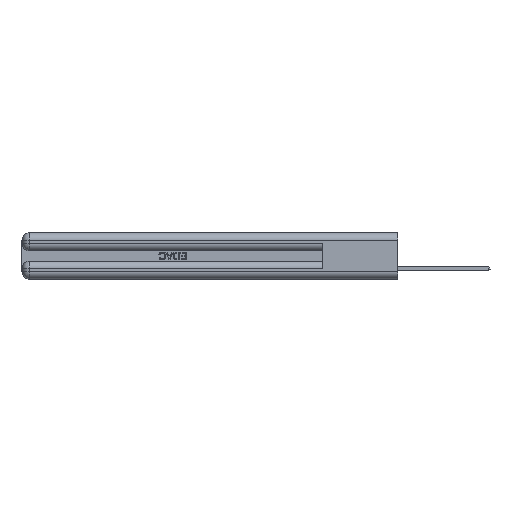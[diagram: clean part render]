
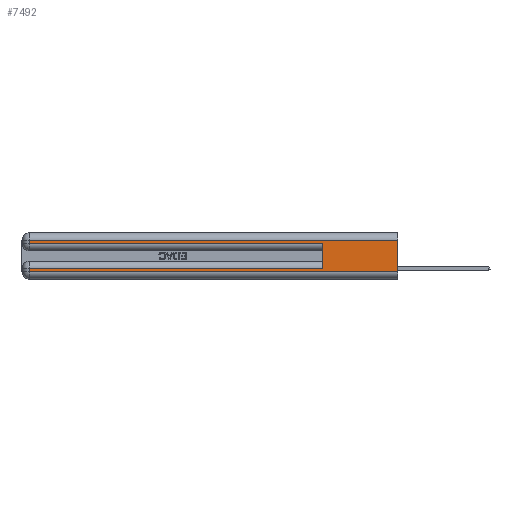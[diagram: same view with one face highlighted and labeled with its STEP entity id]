
A CAD part, left-side view. The second image highlights one B-rep face of the part: STEP entity #7492.
In plain terms, the highlighted planar face has unit normal (-1, 0, 0).
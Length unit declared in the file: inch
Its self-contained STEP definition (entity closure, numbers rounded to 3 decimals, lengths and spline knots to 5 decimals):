
#1328 = VERTEX_POINT ( 'NONE', #38254 ) ;
#1911 = VECTOR ( 'NONE', #44881, 39.37008 ) ;
#5257 = EDGE_CURVE ( 'NONE', #1328, #14109, #14674, .T. ) ;
#5522 = VERTEX_POINT ( 'NONE', #23589 ) ;
#5828 = CARTESIAN_POINT ( 'NONE',  ( 0., 2.94, 0.31 ) ) ;
#6140 = CARTESIAN_POINT ( 'NONE',  ( 0., 0., 0.37 ) ) ;
#7248 = LINE ( 'NONE', #36885, #1911 ) ;
#7492 = ADVANCED_FACE ( 'NONE', ( #13577 ), #10854, .F. ) ;
#7686 = LINE ( 'NONE', #51224, #41666 ) ;
#7776 = VERTEX_POINT ( 'NONE', #51697 ) ;
#8434 = ORIENTED_EDGE ( 'NONE', *, *, #53814, .T. ) ;
#10840 = LINE ( 'NONE', #38863, #15516 ) ;
#10854 = PLANE ( 'NONE',  #31321 ) ;
#11121 = CARTESIAN_POINT ( 'NONE',  ( 0., 0., 0.31 ) ) ;
#11753 = ORIENTED_EDGE ( 'NONE', *, *, #25905, .F. ) ;
#13577 = FACE_OUTER_BOUND ( 'NONE', #14585, .T. ) ;
#14109 = VERTEX_POINT ( 'NONE', #25756 ) ;
#14332 = VECTOR ( 'NONE', #20107, 39.37008 ) ;
#14585 = EDGE_LOOP ( 'NONE', ( #11753, #47032, #16410, #8434, #43683, #26335, #26392, #51709 ) ) ;
#14674 = LINE ( 'NONE', #42219, #18711 ) ;
#15516 = VECTOR ( 'NONE', #30175, 39.37008 ) ;
#16410 = ORIENTED_EDGE ( 'NONE', *, *, #35955, .T. ) ;
#18711 = VECTOR ( 'NONE', #28849, 39.37008 ) ;
#20107 = DIRECTION ( 'NONE',  ( 0., 1., 0. ) ) ;
#21126 = VECTOR ( 'NONE', #30723, 39.37008 ) ;
#21949 = EDGE_CURVE ( 'NONE', #5522, #31353, #50923, .T. ) ;
#22140 = CARTESIAN_POINT ( 'NONE',  ( 0., 0., 0.06 ) ) ;
#22474 = LINE ( 'NONE', #22140, #21126 ) ;
#23235 = CARTESIAN_POINT ( 'NONE',  ( 0., 2.94, 0.06 ) ) ;
#23589 = CARTESIAN_POINT ( 'NONE',  ( 0., 0., 0.31 ) ) ;
#23928 = DIRECTION ( 'NONE',  ( 1., 0., 0. ) ) ;
#25288 = DIRECTION ( 'NONE',  ( 0., 0., -1. ) ) ;
#25756 = CARTESIAN_POINT ( 'NONE',  ( 0., 2.94, 0.085 ) ) ;
#25905 = EDGE_CURVE ( 'NONE', #5522, #35526, #33705, .T. ) ;
#26335 = ORIENTED_EDGE ( 'NONE', *, *, #5257, .T. ) ;
#26392 = ORIENTED_EDGE ( 'NONE', *, *, #52669, .T. ) ;
#28421 = CARTESIAN_POINT ( 'NONE',  ( 0., 0., 0.06 ) ) ;
#28849 = DIRECTION ( 'NONE',  ( 0., 1., 0. ) ) ;
#30175 = DIRECTION ( 'NONE',  ( 0., -1., 0. ) ) ;
#30723 = DIRECTION ( 'NONE',  ( 0., -1., 0. ) ) ;
#31321 = AXIS2_PLACEMENT_3D ( 'NONE', #41568, #23928, #47312 ) ;
#31353 = VERTEX_POINT ( 'NONE', #5828 ) ;
#31973 = VERTEX_POINT ( 'NONE', #23235 ) ;
#32733 = DIRECTION ( 'NONE',  ( 0., 0., 1. ) ) ;
#33705 = LINE ( 'NONE', #6140, #44384 ) ;
#33746 = LINE ( 'NONE', #49228, #54985 ) ;
#35526 = VERTEX_POINT ( 'NONE', #28421 ) ;
#35955 = EDGE_CURVE ( 'NONE', #31353, #7776, #7248, .T. ) ;
#36622 = VERTEX_POINT ( 'NONE', #45545 ) ;
#36885 = CARTESIAN_POINT ( 'NONE',  ( 0., 2.94, 0.37 ) ) ;
#38254 = CARTESIAN_POINT ( 'NONE',  ( 0., 0.6, 0.085 ) ) ;
#38863 = CARTESIAN_POINT ( 'NONE',  ( 0., 0., 0.285 ) ) ;
#39271 = EDGE_CURVE ( 'NONE', #31973, #35526, #22474, .T. ) ;
#39533 = EDGE_CURVE ( 'NONE', #1328, #36622, #33746, .T. ) ;
#41568 = CARTESIAN_POINT ( 'NONE',  ( 0., 0., 0.37 ) ) ;
#41666 = VECTOR ( 'NONE', #25288, 39.37008 ) ;
#42219 = CARTESIAN_POINT ( 'NONE',  ( 0., 0., 0.085 ) ) ;
#43683 = ORIENTED_EDGE ( 'NONE', *, *, #39533, .F. ) ;
#44384 = VECTOR ( 'NONE', #48205, 39.37008 ) ;
#44881 = DIRECTION ( 'NONE',  ( 0., 0., -1. ) ) ;
#45545 = CARTESIAN_POINT ( 'NONE',  ( 0., 0.6, 0.285 ) ) ;
#47032 = ORIENTED_EDGE ( 'NONE', *, *, #21949, .T. ) ;
#47312 = DIRECTION ( 'NONE',  ( 0., 0., -1. ) ) ;
#48205 = DIRECTION ( 'NONE',  ( 0., 0., -1. ) ) ;
#49228 = CARTESIAN_POINT ( 'NONE',  ( 0., 0.6, 0.145 ) ) ;
#50923 = LINE ( 'NONE', #11121, #14332 ) ;
#51224 = CARTESIAN_POINT ( 'NONE',  ( 0., 2.94, 0.37 ) ) ;
#51697 = CARTESIAN_POINT ( 'NONE',  ( 0., 2.94, 0.285 ) ) ;
#51709 = ORIENTED_EDGE ( 'NONE', *, *, #39271, .T. ) ;
#52669 = EDGE_CURVE ( 'NONE', #14109, #31973, #7686, .T. ) ;
#53814 = EDGE_CURVE ( 'NONE', #7776, #36622, #10840, .T. ) ;
#54985 = VECTOR ( 'NONE', #32733, 39.37008 ) ;
